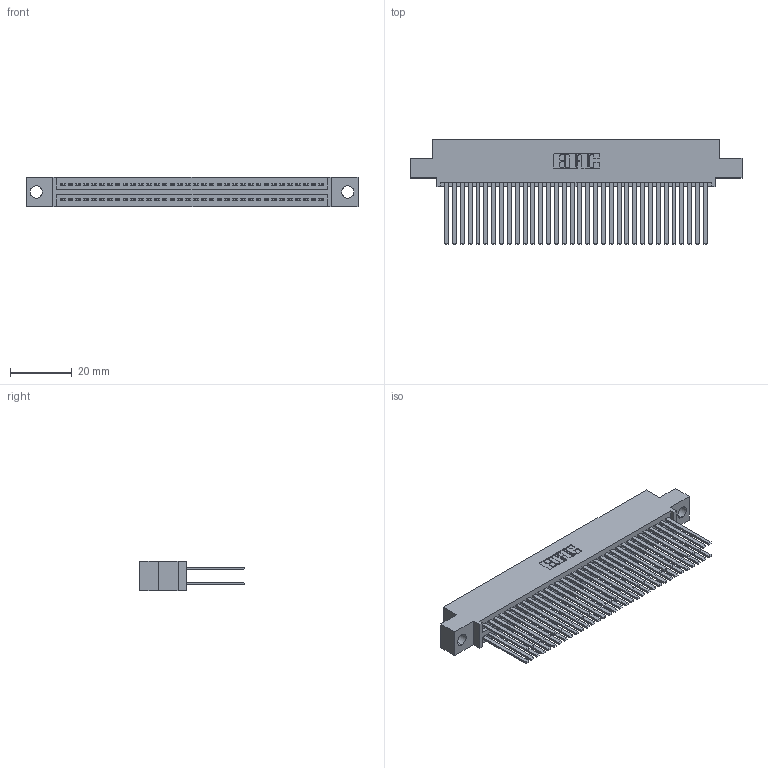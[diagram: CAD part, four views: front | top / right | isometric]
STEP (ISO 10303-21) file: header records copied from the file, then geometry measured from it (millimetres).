
FILE_DESCRIPTION (( 'STEP AP203' ), '1' );
FILE_NAME ('345-068-544-504.STEP', '2018-09-30T13:54:54', ( '' ), ( '' ), 'SwSTEP 2.0', 'SolidWorks 2016', '' );
FILE_SCHEMA (( 'CONFIG_CONTROL_DESIGN' ));
Length unit declared in the file: inch
Products named in the file (3): 345 Part_0.110 Offset - 0.156 Dia-TH; 345-292-001_345-293-144; 345-068-544-504
Assembly tree (69 placements, depth 2):
  345-068-544-504
    345 Part_0.110 Offset - 0.156 Dia-TH
    345-292-001_345-293-144  x68
Bounding box: 107.57 x 33.96 x 9.4 mm (x, y, z)
Volume: 11167.1 mm3; surface area: 19053.8 mm2
Topology: 69 solids, 69 shells, 3122 faces, 9261 edges, 6082 vertices
Faces by surface type: plane 2056, cylinder 1066
Entity records: 27705 total; most frequent: CARTESIAN_POINT 4652, ORIENTED_EDGE 4586, DIRECTION 4109, EDGE_CURVE 2293, LINE 2029, VECTOR 2029, VERTEX_POINT 1526, AXIS2_PLACEMENT_3D 1040
